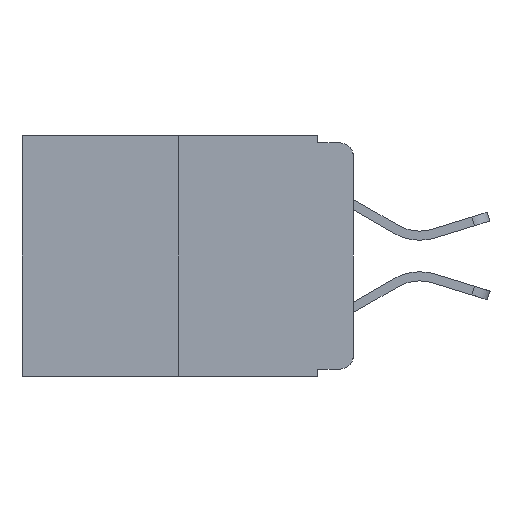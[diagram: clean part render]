
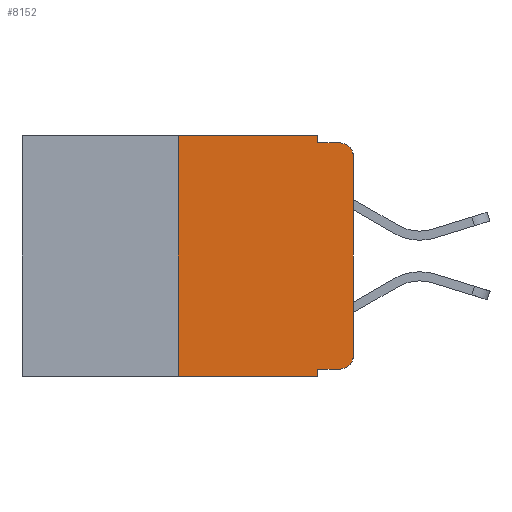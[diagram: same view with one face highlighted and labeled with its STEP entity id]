
A CAD part, left-side view. The second image highlights one B-rep face of the part: STEP entity #8152.
In plain terms, the highlighted planar face has unit normal (-1, 0, 0).
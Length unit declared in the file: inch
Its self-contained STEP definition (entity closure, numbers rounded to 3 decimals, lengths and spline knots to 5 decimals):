
#10 = ORIENTED_EDGE ( 'NONE', *, *, #4925, .F. ) ;
#12 = DIRECTION ( 'NONE',  ( 0., -1., 0. ) ) ;
#83 = DIRECTION ( 'NONE',  ( 0., 0., -1. ) ) ;
#387 = CARTESIAN_POINT ( 'NONE',  ( 0., 0.02, -0.01 ) ) ;
#1075 = FACE_OUTER_BOUND ( 'NONE', #10850, .T. ) ;
#1095 = CARTESIAN_POINT ( 'NONE',  ( 0., 0.02, -0.03 ) ) ;
#1146 = AXIS2_PLACEMENT_3D ( 'NONE', #1095, #9155, #83 ) ;
#1365 = ORIENTED_EDGE ( 'NONE', *, *, #8667, .T. ) ;
#1604 = LINE ( 'NONE', #11444, #3039 ) ;
#1651 = VERTEX_POINT ( 'NONE', #11613 ) ;
#1677 = VECTOR ( 'NONE', #4579, 39.37008 ) ;
#1769 = CARTESIAN_POINT ( 'NONE',  ( 0., 0.473, 0. ) ) ;
#1830 = CARTESIAN_POINT ( 'NONE',  ( 0., 0.25, 0. ) ) ;
#1862 = EDGE_CURVE ( 'NONE', #10209, #11512, #7895, .T. ) ;
#2152 = VERTEX_POINT ( 'NONE', #4858 ) ;
#2219 = DIRECTION ( 'NONE',  ( 0., 0., -1. ) ) ;
#2294 = CARTESIAN_POINT ( 'NONE',  ( 0., 0.051, -0.343 ) ) ;
#2362 = ORIENTED_EDGE ( 'NONE', *, *, #10342, .F. ) ;
#2395 = VECTOR ( 'NONE', #5003, 39.37008 ) ;
#3039 = VECTOR ( 'NONE', #5967, 39.37008 ) ;
#3046 = CARTESIAN_POINT ( 'NONE',  ( 0., 0.051, -0.01 ) ) ;
#3098 = CARTESIAN_POINT ( 'NONE',  ( 0., 0.051, 0. ) ) ;
#3274 = CARTESIAN_POINT ( 'NONE',  ( 0., 0., -0.03 ) ) ;
#3276 = VERTEX_POINT ( 'NONE', #1830 ) ;
#3474 = LINE ( 'NONE', #10137, #9075 ) ;
#3497 = VERTEX_POINT ( 'NONE', #5396 ) ;
#3884 = DIRECTION ( 'NONE',  ( 1., 0., 0. ) ) ;
#3905 = ORIENTED_EDGE ( 'NONE', *, *, #9463, .T. ) ;
#3958 = DIRECTION ( 'NONE',  ( 0., -1., 0. ) ) ;
#4231 = EDGE_CURVE ( 'NONE', #3276, #6601, #4962, .T. ) ;
#4270 = LINE ( 'NONE', #3046, #11306 ) ;
#4341 = CARTESIAN_POINT ( 'NONE',  ( 0., 0.25, 0. ) ) ;
#4579 = DIRECTION ( 'NONE',  ( 0., -1., 0. ) ) ;
#4819 = LINE ( 'NONE', #10484, #2395 ) ;
#4858 = CARTESIAN_POINT ( 'NONE',  ( 0., 0.051, -0.01 ) ) ;
#4907 = VERTEX_POINT ( 'NONE', #9324 ) ;
#4925 = EDGE_CURVE ( 'NONE', #2152, #11512, #4270, .T. ) ;
#4962 = LINE ( 'NONE', #1769, #1677 ) ;
#4975 = CIRCLE ( 'NONE', #11461, 0.02 ) ;
#5003 = DIRECTION ( 'NONE',  ( 0., 0., -1. ) ) ;
#5119 = VECTOR ( 'NONE', #11711, 39.37008 ) ;
#5319 = AXIS2_PLACEMENT_3D ( 'NONE', #6804, #3884, #2219 ) ;
#5396 = CARTESIAN_POINT ( 'NONE',  ( 0., 0., -0.313 ) ) ;
#5460 = CARTESIAN_POINT ( 'NONE',  ( 0., 0.051, 0. ) ) ;
#5462 = ORIENTED_EDGE ( 'NONE', *, *, #6360, .T. ) ;
#5557 = LINE ( 'NONE', #3098, #7426 ) ;
#5717 = CARTESIAN_POINT ( 'NONE',  ( 0., 0.473, -0.343 ) ) ;
#5896 = EDGE_CURVE ( 'NONE', #6447, #3276, #9004, .T. ) ;
#5967 = DIRECTION ( 'NONE',  ( 0., 0., 1. ) ) ;
#6282 = VERTEX_POINT ( 'NONE', #2294 ) ;
#6313 = EDGE_CURVE ( 'NONE', #6601, #2152, #4819, .T. ) ;
#6360 = EDGE_CURVE ( 'NONE', #4907, #3497, #4975, .T. ) ;
#6447 = VERTEX_POINT ( 'NONE', #11542 ) ;
#6601 = VERTEX_POINT ( 'NONE', #5460 ) ;
#6719 = LINE ( 'NONE', #5717, #11331 ) ;
#6804 = CARTESIAN_POINT ( 'NONE',  ( 0., 0.473, 0. ) ) ;
#7318 = ORIENTED_EDGE ( 'NONE', *, *, #6313, .F. ) ;
#7418 = ORIENTED_EDGE ( 'NONE', *, *, #1862, .T. ) ;
#7426 = VECTOR ( 'NONE', #7533, 39.37008 ) ;
#7533 = DIRECTION ( 'NONE',  ( 0., 0., -1. ) ) ;
#7599 = ORIENTED_EDGE ( 'NONE', *, *, #5896, .F. ) ;
#7610 = PLANE ( 'NONE',  #5319 ) ;
#7856 = ORIENTED_EDGE ( 'NONE', *, *, #10012, .T. ) ;
#7895 = CIRCLE ( 'NONE', #1146, 0.02 ) ;
#8051 = CARTESIAN_POINT ( 'NONE',  ( 0., 0.02, -0.313 ) ) ;
#8152 = ADVANCED_FACE ( 'NONE', ( #1075 ), #7610, .F. ) ;
#8667 = EDGE_CURVE ( 'NONE', #1651, #4907, #3474, .T. ) ;
#8668 = ORIENTED_EDGE ( 'NONE', *, *, #4231, .F. ) ;
#8829 = DIRECTION ( 'NONE',  ( 0., 0., -1. ) ) ;
#9004 = LINE ( 'NONE', #4341, #5119 ) ;
#9075 = VECTOR ( 'NONE', #12, 39.37008 ) ;
#9155 = DIRECTION ( 'NONE',  ( -1., 0., 0. ) ) ;
#9324 = CARTESIAN_POINT ( 'NONE',  ( 0., 0.02, -0.333 ) ) ;
#9463 = EDGE_CURVE ( 'NONE', #3497, #10209, #1604, .T. ) ;
#10012 = EDGE_CURVE ( 'NONE', #6447, #6282, #6719, .T. ) ;
#10137 = CARTESIAN_POINT ( 'NONE',  ( 0., 0.051, -0.333 ) ) ;
#10209 = VERTEX_POINT ( 'NONE', #3274 ) ;
#10342 = EDGE_CURVE ( 'NONE', #1651, #6282, #5557, .T. ) ;
#10484 = CARTESIAN_POINT ( 'NONE',  ( 0., 0.051, 0. ) ) ;
#10748 = DIRECTION ( 'NONE',  ( -1., 0., 0. ) ) ;
#10850 = EDGE_LOOP ( 'NONE', ( #3905, #7418, #10, #7318, #8668, #7599, #7856, #2362, #1365, #5462 ) ) ;
#11306 = VECTOR ( 'NONE', #3958, 39.37008 ) ;
#11315 = DIRECTION ( 'NONE',  ( 0., -1., 0. ) ) ;
#11331 = VECTOR ( 'NONE', #11315, 39.37008 ) ;
#11444 = CARTESIAN_POINT ( 'NONE',  ( 0., 0., 0. ) ) ;
#11461 = AXIS2_PLACEMENT_3D ( 'NONE', #8051, #10748, #8829 ) ;
#11512 = VERTEX_POINT ( 'NONE', #387 ) ;
#11542 = CARTESIAN_POINT ( 'NONE',  ( 0., 0.25, -0.343 ) ) ;
#11613 = CARTESIAN_POINT ( 'NONE',  ( 0., 0.051, -0.333 ) ) ;
#11711 = DIRECTION ( 'NONE',  ( 0., 0., 1. ) ) ;
